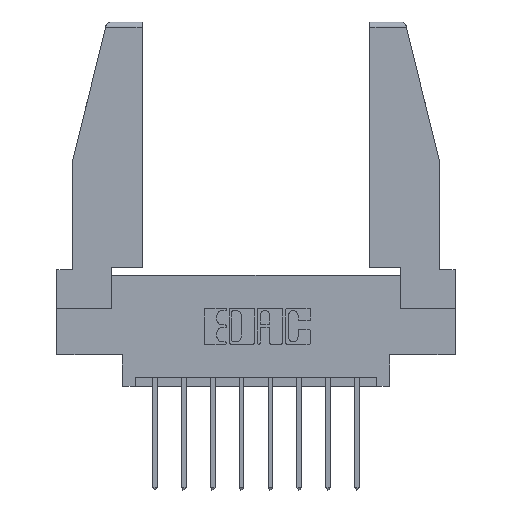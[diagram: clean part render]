
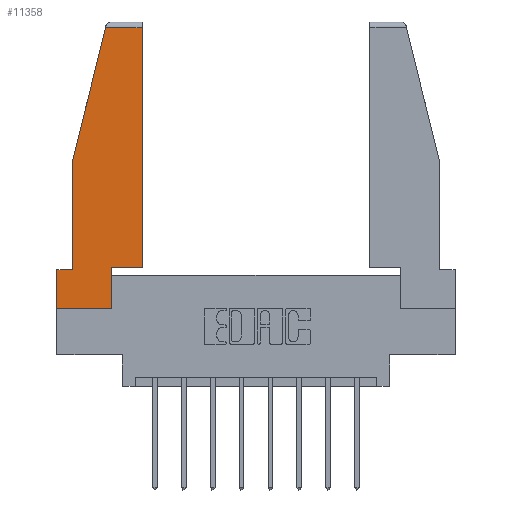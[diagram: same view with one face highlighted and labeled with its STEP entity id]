
A CAD part, top view. The second image highlights one B-rep face of the part: STEP entity #11358.
In plain terms, the highlighted planar face has unit normal (0, 0, 1).
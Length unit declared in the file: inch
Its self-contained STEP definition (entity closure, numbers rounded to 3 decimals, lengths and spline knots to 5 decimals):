
#568 = LINE ( 'NONE', #6125, #5817 ) ;
#1599 = LINE ( 'NONE', #6335, #10211 ) ;
#1728 = EDGE_CURVE ( 'NONE', #10409, #2762, #1599, .T. ) ;
#1742 = DIRECTION ( 'NONE',  ( -0.239, -0.971, 0. ) ) ;
#1972 = DIRECTION ( 'NONE',  ( 0., 1., 0. ) ) ;
#2175 = EDGE_CURVE ( 'NONE', #10581, #8566, #7511, .T. ) ;
#2275 = CARTESIAN_POINT ( 'NONE',  ( 0.086, 0.8, 0. ) ) ;
#2330 = CARTESIAN_POINT ( 'NONE',  ( 0.461, 0.223, 0. ) ) ;
#2762 = VERTEX_POINT ( 'NONE', #7947 ) ;
#2931 = VERTEX_POINT ( 'NONE', #3162 ) ;
#3081 = PLANE ( 'NONE',  #3399 ) ;
#3162 = CARTESIAN_POINT ( 'NONE',  ( 0.461, 1.52, 0. ) ) ;
#3257 = EDGE_CURVE ( 'NONE', #6325, #7706, #7302, .T. ) ;
#3333 = ORIENTED_EDGE ( 'NONE', *, *, #6095, .T. ) ;
#3399 = AXIS2_PLACEMENT_3D ( 'NONE', #10245, #4087, #11279 ) ;
#3493 = VECTOR ( 'NONE', #1972, 39.37008 ) ;
#3949 = VECTOR ( 'NONE', #3968, 39.37008 ) ;
#3968 = DIRECTION ( 'NONE',  ( -1., 0., 0. ) ) ;
#4087 = DIRECTION ( 'NONE',  ( 0., 0., 1. ) ) ;
#4194 = DIRECTION ( 'NONE',  ( 0., 1., 0. ) ) ;
#4258 = CARTESIAN_POINT ( 'NONE',  ( 0.086, 0.21, 0. ) ) ;
#4442 = ORIENTED_EDGE ( 'NONE', *, *, #8328, .T. ) ;
#4526 = FACE_OUTER_BOUND ( 'NONE', #13214, .T. ) ;
#4813 = ORIENTED_EDGE ( 'NONE', *, *, #2175, .T. ) ;
#4947 = CARTESIAN_POINT ( 'NONE',  ( 0.086, 0.8, 0. ) ) ;
#5013 = VECTOR ( 'NONE', #9955, 39.37008 ) ;
#5792 = CARTESIAN_POINT ( 'NONE',  ( 0.297, 0.223, 0. ) ) ;
#5817 = VECTOR ( 'NONE', #9047, 39.37008 ) ;
#5976 = ORIENTED_EDGE ( 'NONE', *, *, #7458, .T. ) ;
#6095 = EDGE_CURVE ( 'NONE', #7706, #10409, #568, .T. ) ;
#6125 = CARTESIAN_POINT ( 'NONE',  ( 0., 0., 0. ) ) ;
#6325 = VERTEX_POINT ( 'NONE', #10454 ) ;
#6327 = VERTEX_POINT ( 'NONE', #4258 ) ;
#6335 = CARTESIAN_POINT ( 'NONE',  ( 0.297, 0., 0. ) ) ;
#7021 = VECTOR ( 'NONE', #1742, 39.37008 ) ;
#7115 = LINE ( 'NONE', #9020, #11912 ) ;
#7302 = LINE ( 'NONE', #10588, #9707 ) ;
#7458 = EDGE_CURVE ( 'NONE', #2762, #7768, #9146, .T. ) ;
#7511 = LINE ( 'NONE', #8956, #7021 ) ;
#7706 = VERTEX_POINT ( 'NONE', #12097 ) ;
#7768 = VERTEX_POINT ( 'NONE', #2330 ) ;
#7947 = CARTESIAN_POINT ( 'NONE',  ( 0.297, 0.223, 0. ) ) ;
#8002 = DIRECTION ( 'NONE',  ( -1., 0., 0. ) ) ;
#8328 = EDGE_CURVE ( 'NONE', #7768, #2931, #12432, .T. ) ;
#8566 = VERTEX_POINT ( 'NONE', #2275 ) ;
#8939 = ORIENTED_EDGE ( 'NONE', *, *, #11759, .T. ) ;
#8956 = CARTESIAN_POINT ( 'NONE',  ( 0.271, 1.55, 0. ) ) ;
#8986 = ORIENTED_EDGE ( 'NONE', *, *, #10840, .T. ) ;
#9020 = CARTESIAN_POINT ( 'NONE',  ( 0., 1.52, 0. ) ) ;
#9047 = DIRECTION ( 'NONE',  ( 1., 0., 0. ) ) ;
#9146 = LINE ( 'NONE', #5792, #9943 ) ;
#9628 = EDGE_CURVE ( 'NONE', #6327, #6325, #10374, .T. ) ;
#9702 = LINE ( 'NONE', #4947, #5013 ) ;
#9707 = VECTOR ( 'NONE', #11633, 39.37008 ) ;
#9798 = CARTESIAN_POINT ( 'NONE',  ( 0.297, 0., 0. ) ) ;
#9828 = DIRECTION ( 'NONE',  ( 1., 0., 0. ) ) ;
#9943 = VECTOR ( 'NONE', #9828, 39.37008 ) ;
#9955 = DIRECTION ( 'NONE',  ( 0., -1., 0. ) ) ;
#10130 = CARTESIAN_POINT ( 'NONE',  ( 0., 0.21, 0. ) ) ;
#10211 = VECTOR ( 'NONE', #4194, 39.37008 ) ;
#10245 = CARTESIAN_POINT ( 'NONE',  ( 0., 0., 0. ) ) ;
#10374 = LINE ( 'NONE', #10130, #3949 ) ;
#10409 = VERTEX_POINT ( 'NONE', #9798 ) ;
#10454 = CARTESIAN_POINT ( 'NONE',  ( 0., 0.21, 0. ) ) ;
#10581 = VERTEX_POINT ( 'NONE', #12078 ) ;
#10588 = CARTESIAN_POINT ( 'NONE',  ( 0., 0.21, 0. ) ) ;
#10840 = EDGE_CURVE ( 'NONE', #8566, #6327, #9702, .T. ) ;
#11275 = CARTESIAN_POINT ( 'NONE',  ( 0.461, 0.223, 0. ) ) ;
#11279 = DIRECTION ( 'NONE',  ( 1., 0., 0. ) ) ;
#11358 = ADVANCED_FACE ( 'NONE', ( #4526 ), #3081, .T. ) ;
#11552 = ORIENTED_EDGE ( 'NONE', *, *, #1728, .T. ) ;
#11633 = DIRECTION ( 'NONE',  ( 0., -1., 0. ) ) ;
#11759 = EDGE_CURVE ( 'NONE', #2931, #10581, #7115, .T. ) ;
#11912 = VECTOR ( 'NONE', #8002, 39.37008 ) ;
#12078 = CARTESIAN_POINT ( 'NONE',  ( 0.2636, 1.52, 0. ) ) ;
#12097 = CARTESIAN_POINT ( 'NONE',  ( 0., 0., 0. ) ) ;
#12432 = LINE ( 'NONE', #11275, #3493 ) ;
#12438 = ORIENTED_EDGE ( 'NONE', *, *, #9628, .T. ) ;
#12454 = ORIENTED_EDGE ( 'NONE', *, *, #3257, .T. ) ;
#13214 = EDGE_LOOP ( 'NONE', ( #4442, #8939, #4813, #8986, #12438, #12454, #3333, #11552, #5976 ) ) ;
